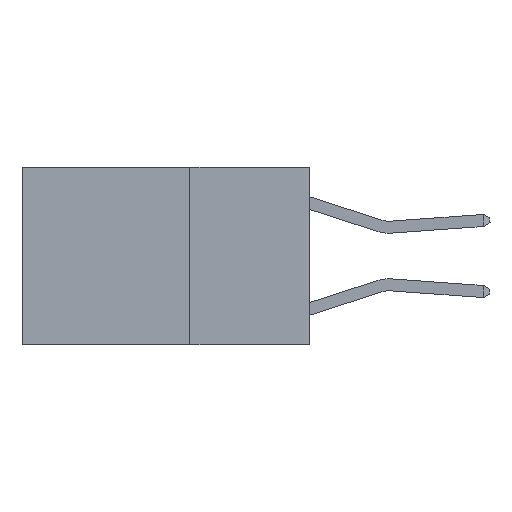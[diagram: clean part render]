
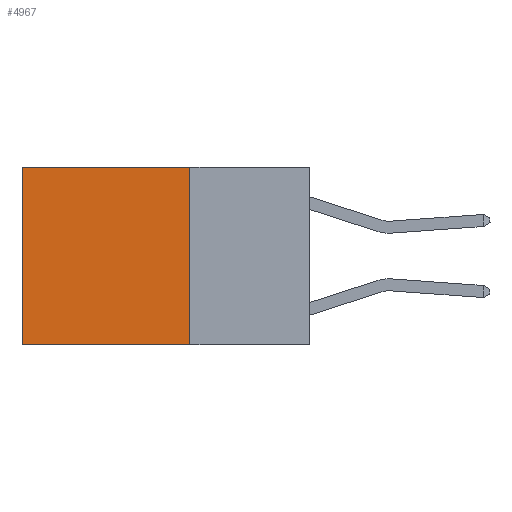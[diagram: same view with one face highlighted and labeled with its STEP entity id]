
A CAD part, left-side view. The second image highlights one B-rep face of the part: STEP entity #4967.
In plain terms, the highlighted planar face has unit normal (-1, 0, 0).
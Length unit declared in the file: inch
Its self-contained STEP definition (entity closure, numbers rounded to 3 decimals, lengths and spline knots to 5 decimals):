
#205 = LINE ( 'NONE', #5735, #2840 ) ;
#793 = EDGE_CURVE ( 'NONE', #12867, #7454, #1939, .T. ) ;
#1330 = VERTEX_POINT ( 'NONE', #6865 ) ;
#1629 = VECTOR ( 'NONE', #10806, 39.37008 ) ;
#1939 = LINE ( 'NONE', #10761, #1629 ) ;
#2503 = DIRECTION ( 'NONE',  ( 0., 0., -1. ) ) ;
#2840 = VECTOR ( 'NONE', #12773, 39.37008 ) ;
#3021 = ORIENTED_EDGE ( 'NONE', *, *, #793, .T. ) ;
#3376 = AXIS2_PLACEMENT_3D ( 'NONE', #5483, #8730, #2503 ) ;
#4567 = EDGE_CURVE ( 'NONE', #5140, #7454, #10585, .T. ) ;
#4956 = CARTESIAN_POINT ( 'NONE',  ( 0.2625, 0.25, -0.37 ) ) ;
#4967 = ADVANCED_FACE ( 'NONE', ( #9600 ), #7697, .F. ) ;
#5031 = EDGE_CURVE ( 'NONE', #1330, #12867, #205, .T. ) ;
#5140 = VERTEX_POINT ( 'NONE', #4956 ) ;
#5483 = CARTESIAN_POINT ( 'NONE',  ( 0.2625, 0.25, 0. ) ) ;
#5735 = CARTESIAN_POINT ( 'NONE',  ( 0.2625, 0.25, 0. ) ) ;
#5745 = ORIENTED_EDGE ( 'NONE', *, *, #4567, .F. ) ;
#6100 = ORIENTED_EDGE ( 'NONE', *, *, #5031, .T. ) ;
#6865 = CARTESIAN_POINT ( 'NONE',  ( 0.2625, 0.25, 0. ) ) ;
#7099 = DIRECTION ( 'NONE',  ( 0., 1., 0. ) ) ;
#7307 = EDGE_CURVE ( 'NONE', #1330, #5140, #8793, .T. ) ;
#7454 = VERTEX_POINT ( 'NONE', #12108 ) ;
#7697 = PLANE ( 'NONE',  #3376 ) ;
#8486 = VECTOR ( 'NONE', #10682, 39.37008 ) ;
#8593 = ORIENTED_EDGE ( 'NONE', *, *, #7307, .F. ) ;
#8730 = DIRECTION ( 'NONE',  ( 1., 0., 0. ) ) ;
#8793 = LINE ( 'NONE', #10724, #8486 ) ;
#9600 = FACE_OUTER_BOUND ( 'NONE', #12101, .T. ) ;
#10064 = CARTESIAN_POINT ( 'NONE',  ( 0.2625, 0.25, -0.37 ) ) ;
#10273 = VECTOR ( 'NONE', #7099, 39.37008 ) ;
#10297 = CARTESIAN_POINT ( 'NONE',  ( 0.2625, 0.6, 0. ) ) ;
#10585 = LINE ( 'NONE', #10064, #10273 ) ;
#10682 = DIRECTION ( 'NONE',  ( 0., 0., -1. ) ) ;
#10724 = CARTESIAN_POINT ( 'NONE',  ( 0.2625, 0.25, 0. ) ) ;
#10761 = CARTESIAN_POINT ( 'NONE',  ( 0.2625, 0.6, 0. ) ) ;
#10806 = DIRECTION ( 'NONE',  ( 0., 0., -1. ) ) ;
#12101 = EDGE_LOOP ( 'NONE', ( #3021, #5745, #8593, #6100 ) ) ;
#12108 = CARTESIAN_POINT ( 'NONE',  ( 0.2625, 0.6, -0.37 ) ) ;
#12773 = DIRECTION ( 'NONE',  ( 0., 1., 0. ) ) ;
#12867 = VERTEX_POINT ( 'NONE', #10297 ) ;
